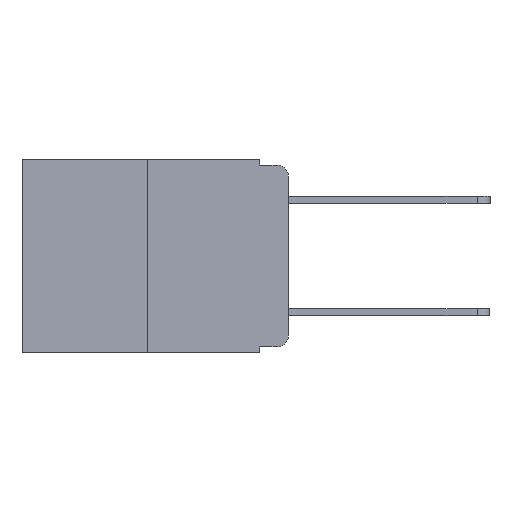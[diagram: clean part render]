
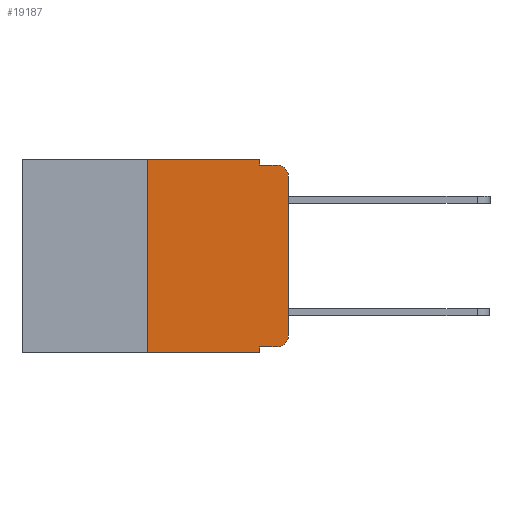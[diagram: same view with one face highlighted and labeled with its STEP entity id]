
A CAD part, left-side view. The second image highlights one B-rep face of the part: STEP entity #19187.
In plain terms, the highlighted planar face has unit normal (-1, 0, 0).
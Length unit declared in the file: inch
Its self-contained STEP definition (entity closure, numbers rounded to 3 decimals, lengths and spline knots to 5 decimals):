
#75 = DIRECTION ( 'NONE',  ( 0., 0., -1. ) ) ;
#221 = DIRECTION ( 'NONE',  ( 0., -1., 0. ) ) ;
#453 = CARTESIAN_POINT ( 'NONE',  ( 0., 0.473, 0. ) ) ;
#478 = CARTESIAN_POINT ( 'NONE',  ( 0., 0.02, -0.01 ) ) ;
#771 = EDGE_CURVE ( 'NONE', #19164, #15984, #11460, .T. ) ;
#784 = CARTESIAN_POINT ( 'NONE',  ( 0., 0., -0.313 ) ) ;
#1130 = CARTESIAN_POINT ( 'NONE',  ( 0., 0.051, -0.333 ) ) ;
#1165 = ORIENTED_EDGE ( 'NONE', *, *, #17553, .T. ) ;
#1601 = VERTEX_POINT ( 'NONE', #784 ) ;
#1992 = EDGE_CURVE ( 'NONE', #11377, #11388, #16783, .T. ) ;
#2528 = LINE ( 'NONE', #453, #13848 ) ;
#3043 = VECTOR ( 'NONE', #13853, 39.37008 ) ;
#3140 = EDGE_CURVE ( 'NONE', #17063, #7182, #7431, .T. ) ;
#3176 = EDGE_CURVE ( 'NONE', #11388, #17063, #2528, .T. ) ;
#3200 = CARTESIAN_POINT ( 'NONE',  ( 0., 0.02, -0.313 ) ) ;
#3723 = AXIS2_PLACEMENT_3D ( 'NONE', #10909, #15226, #6459 ) ;
#3980 = ORIENTED_EDGE ( 'NONE', *, *, #4257, .F. ) ;
#4257 = EDGE_CURVE ( 'NONE', #7182, #5530, #17110, .T. ) ;
#4545 = EDGE_CURVE ( 'NONE', #11377, #15984, #6173, .T. ) ;
#4563 = LINE ( 'NONE', #17402, #9305 ) ;
#4877 = DIRECTION ( 'NONE',  ( 0., 0., -1. ) ) ;
#5187 = ORIENTED_EDGE ( 'NONE', *, *, #19375, .T. ) ;
#5230 = ORIENTED_EDGE ( 'NONE', *, *, #7548, .T. ) ;
#5408 = EDGE_CURVE ( 'NONE', #19076, #5530, #14677, .T. ) ;
#5530 = VERTEX_POINT ( 'NONE', #478 ) ;
#5556 = CARTESIAN_POINT ( 'NONE',  ( 0., 0.473, -0.343 ) ) ;
#5572 = LINE ( 'NONE', #10734, #13488 ) ;
#6173 = LINE ( 'NONE', #5556, #13545 ) ;
#6384 = EDGE_LOOP ( 'NONE', ( #5230, #9663, #3980, #7789, #14872, #9887, #8175, #10379, #5187, #1165 ) ) ;
#6459 = DIRECTION ( 'NONE',  ( 0., 0., -1. ) ) ;
#6713 = CARTESIAN_POINT ( 'NONE',  ( 0., 0., -0.03 ) ) ;
#7182 = VERTEX_POINT ( 'NONE', #12579 ) ;
#7242 = DIRECTION ( 'NONE',  ( 0., 0., 1. ) ) ;
#7268 = CARTESIAN_POINT ( 'NONE',  ( 0., 0.25, -0.343 ) ) ;
#7282 = CARTESIAN_POINT ( 'NONE',  ( 0., 0.25, 0. ) ) ;
#7431 = LINE ( 'NONE', #15077, #3043 ) ;
#7548 = EDGE_CURVE ( 'NONE', #1601, #19076, #5572, .T. ) ;
#7789 = ORIENTED_EDGE ( 'NONE', *, *, #3140, .F. ) ;
#8175 = ORIENTED_EDGE ( 'NONE', *, *, #4545, .T. ) ;
#8856 = DIRECTION ( 'NONE',  ( 0., -1., 0. ) ) ;
#9305 = VECTOR ( 'NONE', #8856, 39.37008 ) ;
#9533 = VECTOR ( 'NONE', #221, 39.37008 ) ;
#9547 = FACE_OUTER_BOUND ( 'NONE', #6384, .T. ) ;
#9637 = VECTOR ( 'NONE', #7242, 39.37008 ) ;
#9663 = ORIENTED_EDGE ( 'NONE', *, *, #5408, .T. ) ;
#9695 = DIRECTION ( 'NONE',  ( 0., -1., 0. ) ) ;
#9887 = ORIENTED_EDGE ( 'NONE', *, *, #1992, .F. ) ;
#9981 = DIRECTION ( 'NONE',  ( -1., 0., 0. ) ) ;
#10311 = CARTESIAN_POINT ( 'NONE',  ( 0., 0.25, 0. ) ) ;
#10341 = CIRCLE ( 'NONE', #11274, 0.02 ) ;
#10379 = ORIENTED_EDGE ( 'NONE', *, *, #771, .F. ) ;
#10734 = CARTESIAN_POINT ( 'NONE',  ( 0., 0., 0. ) ) ;
#10909 = CARTESIAN_POINT ( 'NONE',  ( 0., 0.473, 0. ) ) ;
#11274 = AXIS2_PLACEMENT_3D ( 'NONE', #3200, #13912, #4877 ) ;
#11377 = VERTEX_POINT ( 'NONE', #7268 ) ;
#11388 = VERTEX_POINT ( 'NONE', #10311 ) ;
#11460 = LINE ( 'NONE', #14108, #15773 ) ;
#12579 = CARTESIAN_POINT ( 'NONE',  ( 0., 0.051, -0.01 ) ) ;
#12664 = VERTEX_POINT ( 'NONE', #12781 ) ;
#12781 = CARTESIAN_POINT ( 'NONE',  ( 0., 0.02, -0.333 ) ) ;
#13057 = DIRECTION ( 'NONE',  ( 0., -1., 0. ) ) ;
#13488 = VECTOR ( 'NONE', #19143, 39.37008 ) ;
#13545 = VECTOR ( 'NONE', #9695, 39.37008 ) ;
#13577 = DIRECTION ( 'NONE',  ( 0., 0., -1. ) ) ;
#13848 = VECTOR ( 'NONE', #13057, 39.37008 ) ;
#13853 = DIRECTION ( 'NONE',  ( 0., 0., -1. ) ) ;
#13912 = DIRECTION ( 'NONE',  ( -1., 0., 0. ) ) ;
#14108 = CARTESIAN_POINT ( 'NONE',  ( 0., 0.051, 0. ) ) ;
#14677 = CIRCLE ( 'NONE', #15400, 0.02 ) ;
#14872 = ORIENTED_EDGE ( 'NONE', *, *, #3176, .F. ) ;
#15077 = CARTESIAN_POINT ( 'NONE',  ( 0., 0.051, 0. ) ) ;
#15169 = PLANE ( 'NONE',  #3723 ) ;
#15226 = DIRECTION ( 'NONE',  ( 1., 0., 0. ) ) ;
#15400 = AXIS2_PLACEMENT_3D ( 'NONE', #18419, #9981, #75 ) ;
#15773 = VECTOR ( 'NONE', #13577, 39.37008 ) ;
#15876 = CARTESIAN_POINT ( 'NONE',  ( 0., 0.051, 0. ) ) ;
#15984 = VERTEX_POINT ( 'NONE', #19384 ) ;
#16783 = LINE ( 'NONE', #7282, #9637 ) ;
#17063 = VERTEX_POINT ( 'NONE', #15876 ) ;
#17110 = LINE ( 'NONE', #18524, #9533 ) ;
#17402 = CARTESIAN_POINT ( 'NONE',  ( 0., 0.051, -0.333 ) ) ;
#17553 = EDGE_CURVE ( 'NONE', #12664, #1601, #10341, .T. ) ;
#18419 = CARTESIAN_POINT ( 'NONE',  ( 0., 0.02, -0.03 ) ) ;
#18524 = CARTESIAN_POINT ( 'NONE',  ( 0., 0.051, -0.01 ) ) ;
#19076 = VERTEX_POINT ( 'NONE', #6713 ) ;
#19143 = DIRECTION ( 'NONE',  ( 0., 0., 1. ) ) ;
#19164 = VERTEX_POINT ( 'NONE', #1130 ) ;
#19187 = ADVANCED_FACE ( 'NONE', ( #9547 ), #15169, .F. ) ;
#19375 = EDGE_CURVE ( 'NONE', #19164, #12664, #4563, .T. ) ;
#19384 = CARTESIAN_POINT ( 'NONE',  ( 0., 0.051, -0.343 ) ) ;
